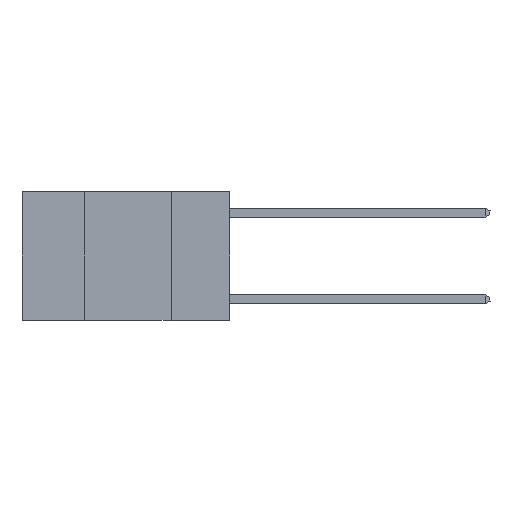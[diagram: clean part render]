
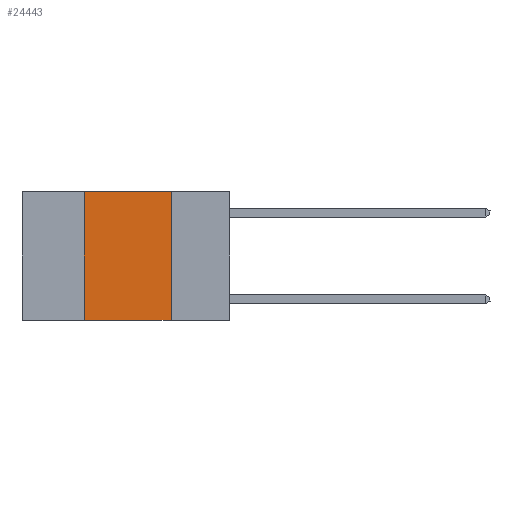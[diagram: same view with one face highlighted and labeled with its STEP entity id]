
A CAD part, left-side view. The second image highlights one B-rep face of the part: STEP entity #24443.
In plain terms, the highlighted planar face has unit normal (-1, 0, 0).
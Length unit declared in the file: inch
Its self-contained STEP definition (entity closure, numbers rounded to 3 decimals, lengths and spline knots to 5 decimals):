
#60 = VERTEX_POINT ( 'NONE', #15221 ) ;
#996 = ORIENTED_EDGE ( 'NONE', *, *, #10660, .F. ) ;
#2037 = DIRECTION ( 'NONE',  ( 0., -1., 0. ) ) ;
#2357 = VERTEX_POINT ( 'NONE', #23553 ) ;
#2547 = AXIS2_PLACEMENT_3D ( 'NONE', #13870, #22571, #17959 ) ;
#3412 = ORIENTED_EDGE ( 'NONE', *, *, #9409, .F. ) ;
#4857 = ORIENTED_EDGE ( 'NONE', *, *, #26615, .F. ) ;
#6518 = LINE ( 'NONE', #15329, #21962 ) ;
#8270 = CARTESIAN_POINT ( 'NONE',  ( 0., 0.42, -0.37 ) ) ;
#9390 = PLANE ( 'NONE',  #2547 ) ;
#9409 = EDGE_CURVE ( 'NONE', #21704, #60, #18081, .T. ) ;
#10660 = EDGE_CURVE ( 'NONE', #2357, #21704, #6518, .T. ) ;
#11803 = EDGE_LOOP ( 'NONE', ( #3412, #996, #4857, #16514 ) ) ;
#11973 = CARTESIAN_POINT ( 'NONE',  ( 0., 0.17, 0. ) ) ;
#12704 = LINE ( 'NONE', #19499, #21211 ) ;
#13870 = CARTESIAN_POINT ( 'NONE',  ( 0., 0.6, 0. ) ) ;
#15221 = CARTESIAN_POINT ( 'NONE',  ( 0., 0.17, -0.37 ) ) ;
#15329 = CARTESIAN_POINT ( 'NONE',  ( 0., 0.6, 0. ) ) ;
#16514 = ORIENTED_EDGE ( 'NONE', *, *, #17238, .T. ) ;
#17238 = EDGE_CURVE ( 'NONE', #19997, #60, #12704, .T. ) ;
#17455 = LINE ( 'NONE', #19341, #27025 ) ;
#17959 = DIRECTION ( 'NONE',  ( 0., 0., -1. ) ) ;
#18081 = LINE ( 'NONE', #26906, #22374 ) ;
#19341 = CARTESIAN_POINT ( 'NONE',  ( 0., 0.42, 0. ) ) ;
#19499 = CARTESIAN_POINT ( 'NONE',  ( 0., 0.6, -0.37 ) ) ;
#19997 = VERTEX_POINT ( 'NONE', #8270 ) ;
#21211 = VECTOR ( 'NONE', #2037, 39.37008 ) ;
#21704 = VERTEX_POINT ( 'NONE', #11973 ) ;
#21791 = DIRECTION ( 'NONE',  ( 0., 0., 1. ) ) ;
#21962 = VECTOR ( 'NONE', #26208, 39.37008 ) ;
#22374 = VECTOR ( 'NONE', #24742, 39.37008 ) ;
#22571 = DIRECTION ( 'NONE',  ( 1., 0., 0. ) ) ;
#23553 = CARTESIAN_POINT ( 'NONE',  ( 0., 0.42, 0. ) ) ;
#24443 = ADVANCED_FACE ( 'NONE', ( #24614 ), #9390, .F. ) ;
#24614 = FACE_OUTER_BOUND ( 'NONE', #11803, .T. ) ;
#24742 = DIRECTION ( 'NONE',  ( 0., 0., -1. ) ) ;
#26208 = DIRECTION ( 'NONE',  ( 0., -1., 0. ) ) ;
#26615 = EDGE_CURVE ( 'NONE', #19997, #2357, #17455, .T. ) ;
#26906 = CARTESIAN_POINT ( 'NONE',  ( 0., 0.17, 0. ) ) ;
#27025 = VECTOR ( 'NONE', #21791, 39.37008 ) ;
